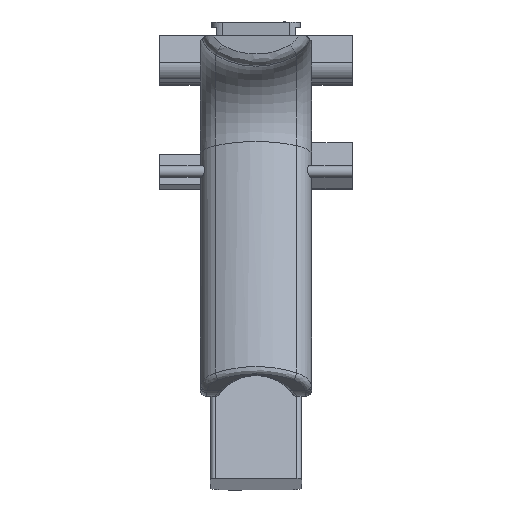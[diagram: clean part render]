
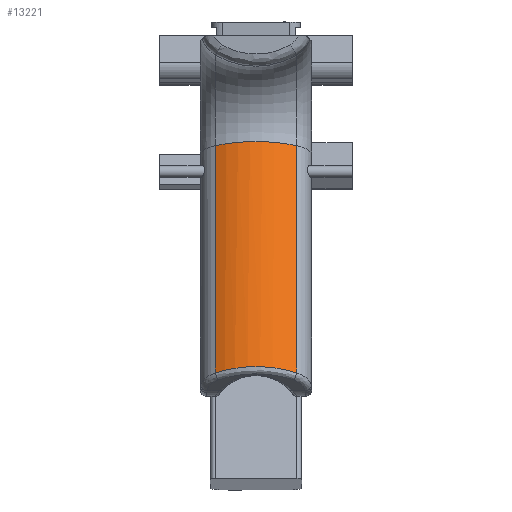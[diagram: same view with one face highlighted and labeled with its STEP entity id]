
A CAD part, left-side view. The second image highlights one B-rep face of the part: STEP entity #13221.
In plain terms, the highlighted cylindrical face has radius 20.552 mm (diameter 41.104 mm), a partial arc.
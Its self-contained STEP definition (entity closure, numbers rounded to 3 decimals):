
#1078=LINE('',#32308,#2059);
#1079=LINE('',#32317,#2060);
#2059=VECTOR('',#16192,10.);
#2060=VECTOR('',#16197,10.);
#2611=CYLINDRICAL_SURFACE('',#14144,20.552);
#2784=ELLIPSE('',#14145,21.05,20.552);
#3175=FACE_OUTER_BOUND('',#3872,.T.);
#3872=EDGE_LOOP('',(#10713,#10714,#10715,#10716));
#4431=CIRCLE('',#14130,20.552);
#5958=VERTEX_POINT('',#32060);
#5964=VERTEX_POINT('',#32110);
#5976=VERTEX_POINT('',#32305);
#5979=VERTEX_POINT('',#32316);
#7686=EDGE_CURVE('',#5964,#5958,#4431,.T.);
#7704=EDGE_CURVE('',#5976,#5958,#1078,.T.);
#7707=EDGE_CURVE('',#5979,#5964,#1079,.T.);
#7708=EDGE_CURVE('',#5979,#5976,#2784,.T.);
#10713=ORIENTED_EDGE('',*,*,#7707,.T.);
#10714=ORIENTED_EDGE('',*,*,#7686,.T.);
#10715=ORIENTED_EDGE('',*,*,#7704,.F.);
#10716=ORIENTED_EDGE('',*,*,#7708,.F.);
#13221=ADVANCED_FACE('',(#3175),#2611,.T.);
#14130=AXIS2_PLACEMENT_3D('',#32158,#16158,#16159);
#14144=AXIS2_PLACEMENT_3D('',#32315,#16195,#16196);
#14145=AXIS2_PLACEMENT_3D('',#32318,#16198,#16199);
#16158=DIRECTION('center_axis',(-0.367,-0.93,0.));
#16159=DIRECTION('ref_axis',(-0.799,0.315,0.512));
#16192=DIRECTION('',(0.367,0.93,0.));
#16195=DIRECTION('center_axis',(0.367,0.93,0.));
#16196=DIRECTION('ref_axis',(-0.799,0.315,0.512));
#16197=DIRECTION('',(0.367,0.93,0.));
#16198=DIRECTION('center_axis',(-0.559,-0.829,0.));
#16199=DIRECTION('ref_axis',(-0.829,0.559,0.));
#32060=CARTESIAN_POINT('',(14.736,-30.517,-10.529));
#32110=CARTESIAN_POINT('',(14.736,-30.517,10.529));
#32158=CARTESIAN_POINT('Origin',(31.157,-36.986,0.));
#32305=CARTESIAN_POINT('',(-8.48,-89.454,-10.529));
#32308=CARTESIAN_POINT('',(-10.338,-94.17,-10.529));
#32315=CARTESIAN_POINT('Origin',(6.084,-100.639,0.));
#32316=CARTESIAN_POINT('',(-8.48,-89.454,10.529));
#32317=CARTESIAN_POINT('',(-10.338,-94.17,10.529));
#32318=CARTESIAN_POINT('Origin',(6.509,-99.56,0.));
